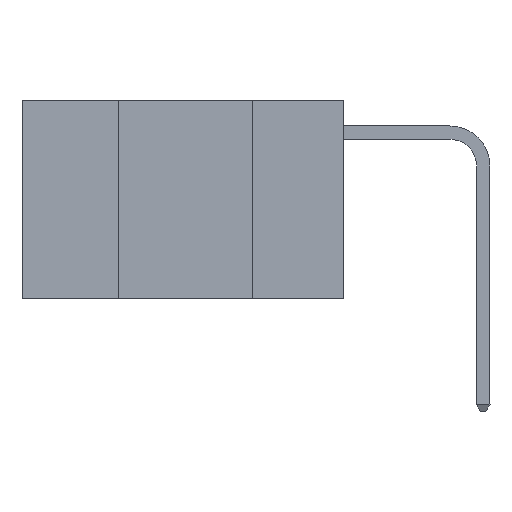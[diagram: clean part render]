
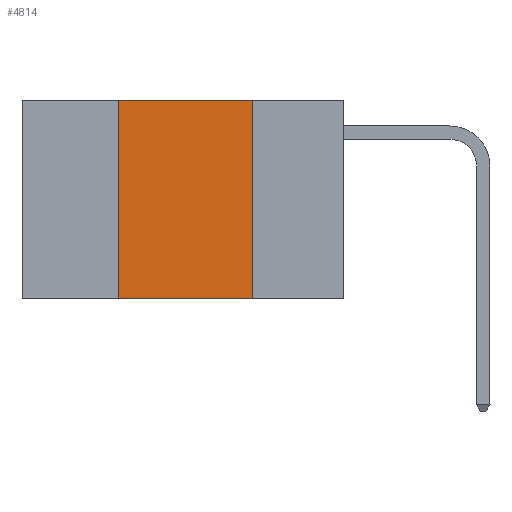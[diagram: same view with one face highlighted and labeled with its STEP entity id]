
A CAD part, left-side view. The second image highlights one B-rep face of the part: STEP entity #4814.
In plain terms, the highlighted planar face has unit normal (-1, 0, 0).
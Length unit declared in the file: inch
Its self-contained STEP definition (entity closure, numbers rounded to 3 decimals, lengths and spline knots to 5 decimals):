
#2 = CARTESIAN_POINT ( 'NONE',  ( 0., 0.6, 0. ) ) ;
#236 = AXIS2_PLACEMENT_3D ( 'NONE', #2, #7512, #11404 ) ;
#335 = ORIENTED_EDGE ( 'NONE', *, *, #11335, .F. ) ;
#510 = CARTESIAN_POINT ( 'NONE',  ( 0., 0.6, -0.37 ) ) ;
#1002 = PLANE ( 'NONE',  #236 ) ;
#2035 = CARTESIAN_POINT ( 'NONE',  ( 0., 0.42, -0.37 ) ) ;
#2368 = LINE ( 'NONE', #7015, #6964 ) ;
#2511 = CARTESIAN_POINT ( 'NONE',  ( 0., 0.42, 0. ) ) ;
#2676 = CARTESIAN_POINT ( 'NONE',  ( 0., 0.42, 0. ) ) ;
#2910 = LINE ( 'NONE', #9212, #9865 ) ;
#3446 = VERTEX_POINT ( 'NONE', #2511 ) ;
#3714 = EDGE_CURVE ( 'NONE', #8581, #6975, #2368, .T. ) ;
#4240 = LINE ( 'NONE', #510, #6724 ) ;
#4814 = ADVANCED_FACE ( 'NONE', ( #9375 ), #1002, .F. ) ;
#6098 = DIRECTION ( 'NONE',  ( 0., 0., -1. ) ) ;
#6227 = DIRECTION ( 'NONE',  ( 0., 0., 1. ) ) ;
#6724 = VECTOR ( 'NONE', #7956, 39.37008 ) ;
#6808 = EDGE_CURVE ( 'NONE', #3446, #8581, #2910, .T. ) ;
#6964 = VECTOR ( 'NONE', #6098, 39.37008 ) ;
#6975 = VERTEX_POINT ( 'NONE', #9505 ) ;
#7015 = CARTESIAN_POINT ( 'NONE',  ( 0., 0.17, 0. ) ) ;
#7067 = EDGE_CURVE ( 'NONE', #10552, #6975, #4240, .T. ) ;
#7361 = VECTOR ( 'NONE', #6227, 39.37008 ) ;
#7512 = DIRECTION ( 'NONE',  ( 1., 0., 0. ) ) ;
#7519 = CARTESIAN_POINT ( 'NONE',  ( 0., 0.17, 0. ) ) ;
#7956 = DIRECTION ( 'NONE',  ( 0., -1., 0. ) ) ;
#8581 = VERTEX_POINT ( 'NONE', #7519 ) ;
#9182 = ORIENTED_EDGE ( 'NONE', *, *, #7067, .T. ) ;
#9212 = CARTESIAN_POINT ( 'NONE',  ( 0., 0.6, 0. ) ) ;
#9375 = FACE_OUTER_BOUND ( 'NONE', #10397, .T. ) ;
#9505 = CARTESIAN_POINT ( 'NONE',  ( 0., 0.17, -0.37 ) ) ;
#9865 = VECTOR ( 'NONE', #10383, 39.37008 ) ;
#10259 = ORIENTED_EDGE ( 'NONE', *, *, #6808, .F. ) ;
#10383 = DIRECTION ( 'NONE',  ( 0., -1., 0. ) ) ;
#10397 = EDGE_LOOP ( 'NONE', ( #11328, #10259, #335, #9182 ) ) ;
#10552 = VERTEX_POINT ( 'NONE', #2035 ) ;
#11089 = LINE ( 'NONE', #2676, #7361 ) ;
#11328 = ORIENTED_EDGE ( 'NONE', *, *, #3714, .F. ) ;
#11335 = EDGE_CURVE ( 'NONE', #10552, #3446, #11089, .T. ) ;
#11404 = DIRECTION ( 'NONE',  ( 0., 0., -1. ) ) ;
